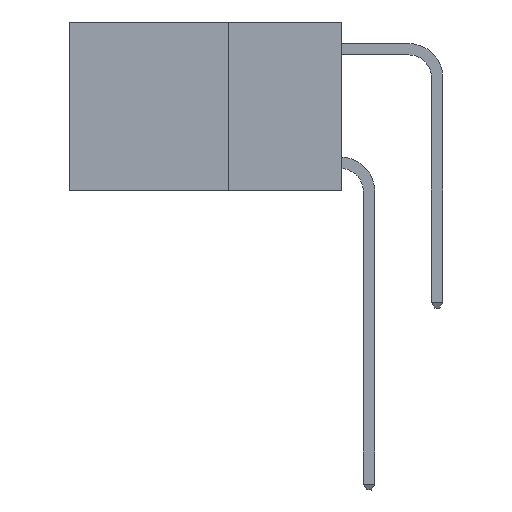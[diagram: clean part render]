
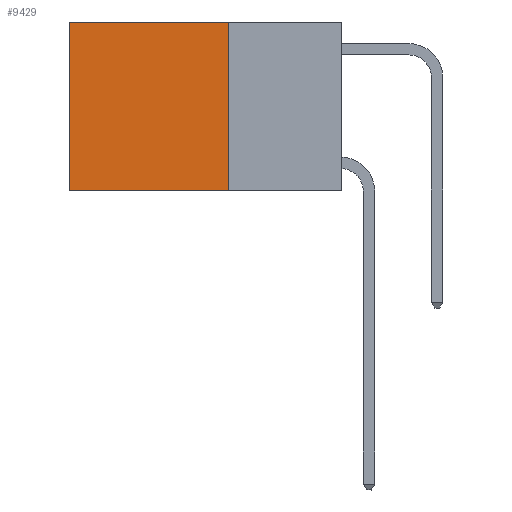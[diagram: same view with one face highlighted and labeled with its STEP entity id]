
A CAD part, left-side view. The second image highlights one B-rep face of the part: STEP entity #9429.
In plain terms, the highlighted planar face has unit normal (-1, 0, 0).
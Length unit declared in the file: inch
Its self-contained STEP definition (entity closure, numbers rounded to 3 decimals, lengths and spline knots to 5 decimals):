
#59 = VECTOR ( 'NONE', #1944, 39.37008 ) ;
#79 = EDGE_CURVE ( 'NONE', #11426, #3040, #3298, .T. ) ;
#961 = ORIENTED_EDGE ( 'NONE', *, *, #8946, .F. ) ;
#997 = VERTEX_POINT ( 'NONE', #1562 ) ;
#1562 = CARTESIAN_POINT ( 'NONE',  ( 0.2625, 0.25, -0.37 ) ) ;
#1944 = DIRECTION ( 'NONE',  ( 0., 1., 0. ) ) ;
#2131 = FACE_OUTER_BOUND ( 'NONE', #2664, .T. ) ;
#2541 = DIRECTION ( 'NONE',  ( 0., 0., -1. ) ) ;
#2664 = EDGE_LOOP ( 'NONE', ( #10946, #4784, #961, #11985 ) ) ;
#2888 = VECTOR ( 'NONE', #10441, 39.37008 ) ;
#3040 = VERTEX_POINT ( 'NONE', #12863 ) ;
#3298 = LINE ( 'NONE', #12715, #7244 ) ;
#3500 = CARTESIAN_POINT ( 'NONE',  ( 0.2625, 0.25, 0. ) ) ;
#4784 = ORIENTED_EDGE ( 'NONE', *, *, #13452, .F. ) ;
#5216 = LINE ( 'NONE', #5937, #2888 ) ;
#5937 = CARTESIAN_POINT ( 'NONE',  ( 0.2625, 0.25, 0. ) ) ;
#7052 = CARTESIAN_POINT ( 'NONE',  ( 0.2625, 0.25, -0.37 ) ) ;
#7244 = VECTOR ( 'NONE', #11521, 39.37008 ) ;
#7887 = CARTESIAN_POINT ( 'NONE',  ( 0.2625, 0.6, -0.37 ) ) ;
#8704 = LINE ( 'NONE', #7052, #59 ) ;
#8946 = EDGE_CURVE ( 'NONE', #11426, #997, #5216, .T. ) ;
#8960 = DIRECTION ( 'NONE',  ( 0., 0., -1. ) ) ;
#9040 = DIRECTION ( 'NONE',  ( 1., 0., 0. ) ) ;
#9133 = VECTOR ( 'NONE', #8960, 39.37008 ) ;
#9429 = ADVANCED_FACE ( 'NONE', ( #2131 ), #14822, .F. ) ;
#9617 = AXIS2_PLACEMENT_3D ( 'NONE', #3500, #9040, #2541 ) ;
#9983 = CARTESIAN_POINT ( 'NONE',  ( 0.2625, 0.6, 0. ) ) ;
#10035 = VERTEX_POINT ( 'NONE', #7887 ) ;
#10441 = DIRECTION ( 'NONE',  ( 0., 0., -1. ) ) ;
#10511 = EDGE_CURVE ( 'NONE', #3040, #10035, #12360, .T. ) ;
#10946 = ORIENTED_EDGE ( 'NONE', *, *, #10511, .T. ) ;
#11426 = VERTEX_POINT ( 'NONE', #14299 ) ;
#11521 = DIRECTION ( 'NONE',  ( 0., 1., 0. ) ) ;
#11985 = ORIENTED_EDGE ( 'NONE', *, *, #79, .T. ) ;
#12360 = LINE ( 'NONE', #9983, #9133 ) ;
#12715 = CARTESIAN_POINT ( 'NONE',  ( 0.2625, 0.25, 0. ) ) ;
#12863 = CARTESIAN_POINT ( 'NONE',  ( 0.2625, 0.6, 0. ) ) ;
#13452 = EDGE_CURVE ( 'NONE', #997, #10035, #8704, .T. ) ;
#14299 = CARTESIAN_POINT ( 'NONE',  ( 0.2625, 0.25, 0. ) ) ;
#14822 = PLANE ( 'NONE',  #9617 ) ;
